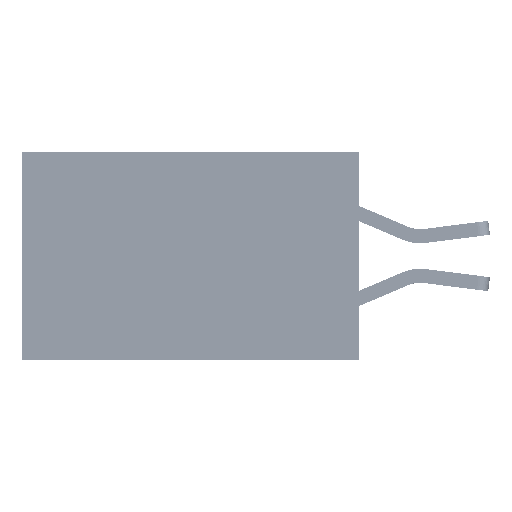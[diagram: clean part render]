
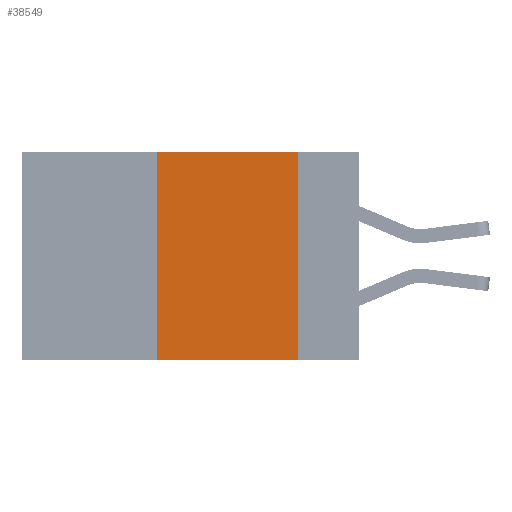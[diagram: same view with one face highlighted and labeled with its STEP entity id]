
A CAD part, left-side view. The second image highlights one B-rep face of the part: STEP entity #38549.
In plain terms, the highlighted planar face has unit normal (-1, 0, 0).
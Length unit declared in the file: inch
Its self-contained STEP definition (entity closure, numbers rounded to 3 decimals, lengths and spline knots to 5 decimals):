
#59 = CARTESIAN_POINT ( 'NONE',  ( 0., 0.6, 0. ) ) ;
#131 = LINE ( 'NONE', #27562, #38154 ) ;
#568 = DIRECTION ( 'NONE',  ( 0., -1., 0. ) ) ;
#1069 = DIRECTION ( 'NONE',  ( 1., 0., 0. ) ) ;
#1299 = DIRECTION ( 'NONE',  ( 0., 0., -1. ) ) ;
#1469 = DIRECTION ( 'NONE',  ( 0., 0., -1. ) ) ;
#1596 = LINE ( 'NONE', #59, #33891 ) ;
#2920 = DIRECTION ( 'NONE',  ( 0., -1., 0. ) ) ;
#4058 = LINE ( 'NONE', #4688, #21872 ) ;
#4688 = CARTESIAN_POINT ( 'NONE',  ( 0., 0.11, 0. ) ) ;
#5577 = ORIENTED_EDGE ( 'NONE', *, *, #24380, .F. ) ;
#5669 = EDGE_LOOP ( 'NONE', ( #23671, #5577, #27620, #18426 ) ) ;
#6587 = EDGE_CURVE ( 'NONE', #24595, #20863, #17913, .T. ) ;
#15547 = EDGE_CURVE ( 'NONE', #24595, #17675, #131, .T. ) ;
#17675 = VERTEX_POINT ( 'NONE', #38301 ) ;
#17913 = LINE ( 'NONE', #21829, #18899 ) ;
#18426 = ORIENTED_EDGE ( 'NONE', *, *, #6587, .T. ) ;
#18899 = VECTOR ( 'NONE', #568, 39.37008 ) ;
#20863 = VERTEX_POINT ( 'NONE', #33642 ) ;
#20934 = AXIS2_PLACEMENT_3D ( 'NONE', #22854, #1069, #1469 ) ;
#21829 = CARTESIAN_POINT ( 'NONE',  ( 0., 0.6, -0.37 ) ) ;
#21872 = VECTOR ( 'NONE', #1299, 39.37008 ) ;
#22205 = PLANE ( 'NONE',  #20934 ) ;
#22369 = VERTEX_POINT ( 'NONE', #31758 ) ;
#22854 = CARTESIAN_POINT ( 'NONE',  ( 0., 0.6, 0. ) ) ;
#23671 = ORIENTED_EDGE ( 'NONE', *, *, #24123, .F. ) ;
#24123 = EDGE_CURVE ( 'NONE', #22369, #20863, #4058, .T. ) ;
#24380 = EDGE_CURVE ( 'NONE', #17675, #22369, #1596, .T. ) ;
#24595 = VERTEX_POINT ( 'NONE', #27913 ) ;
#24857 = DIRECTION ( 'NONE',  ( 0., 0., 1. ) ) ;
#27562 = CARTESIAN_POINT ( 'NONE',  ( 0., 0.36, 0. ) ) ;
#27620 = ORIENTED_EDGE ( 'NONE', *, *, #15547, .F. ) ;
#27913 = CARTESIAN_POINT ( 'NONE',  ( 0., 0.36, -0.37 ) ) ;
#31758 = CARTESIAN_POINT ( 'NONE',  ( 0., 0.11, 0. ) ) ;
#33642 = CARTESIAN_POINT ( 'NONE',  ( 0., 0.11, -0.37 ) ) ;
#33891 = VECTOR ( 'NONE', #2920, 39.37008 ) ;
#38154 = VECTOR ( 'NONE', #24857, 39.37008 ) ;
#38301 = CARTESIAN_POINT ( 'NONE',  ( 0., 0.36, 0. ) ) ;
#38549 = ADVANCED_FACE ( 'NONE', ( #38640 ), #22205, .F. ) ;
#38640 = FACE_OUTER_BOUND ( 'NONE', #5669, .T. ) ;
